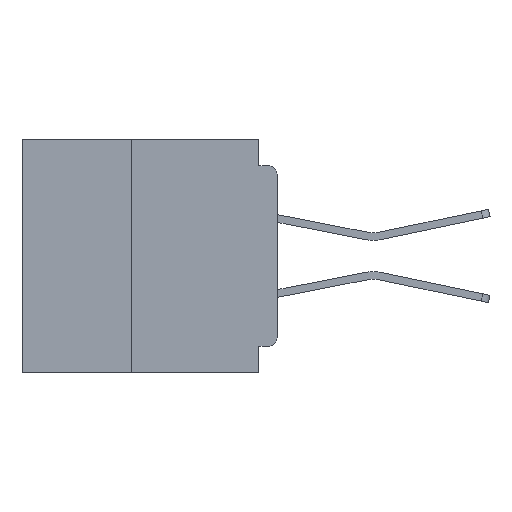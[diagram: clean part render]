
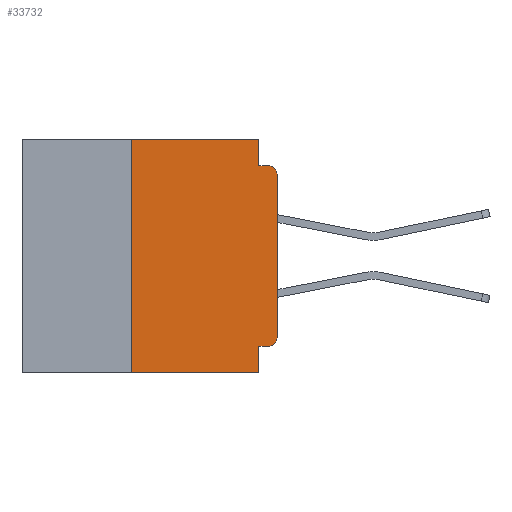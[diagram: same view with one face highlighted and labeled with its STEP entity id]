
A CAD part, left-side view. The second image highlights one B-rep face of the part: STEP entity #33732.
In plain terms, the highlighted planar face has unit normal (-1, 0, 0).
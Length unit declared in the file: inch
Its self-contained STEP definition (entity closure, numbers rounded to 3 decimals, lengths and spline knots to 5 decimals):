
#465 = CARTESIAN_POINT ( 'NONE',  ( 0., 0.437, -0.4 ) ) ;
#1967 = PLANE ( 'NONE',  #48485 ) ;
#2729 = VECTOR ( 'NONE', #35786, 39.37008 ) ;
#2895 = VECTOR ( 'NONE', #12033, 39.37008 ) ;
#3244 = VERTEX_POINT ( 'NONE', #47638 ) ;
#3533 = ORIENTED_EDGE ( 'NONE', *, *, #6978, .F. ) ;
#4077 = LINE ( 'NONE', #23876, #15611 ) ;
#4871 = VECTOR ( 'NONE', #42833, 39.37008 ) ;
#4884 = AXIS2_PLACEMENT_3D ( 'NONE', #11388, #45595, #16334 ) ;
#5886 = ORIENTED_EDGE ( 'NONE', *, *, #40494, .T. ) ;
#6628 = ORIENTED_EDGE ( 'NONE', *, *, #50341, .T. ) ;
#6978 = EDGE_CURVE ( 'NONE', #46135, #61625, #45767, .T. ) ;
#9293 = EDGE_CURVE ( 'NONE', #43562, #58347, #61376, .T. ) ;
#10098 = ORIENTED_EDGE ( 'NONE', *, *, #47548, .F. ) ;
#10456 = CARTESIAN_POINT ( 'NONE',  ( 0., 0.015, -0.06 ) ) ;
#11388 = CARTESIAN_POINT ( 'NONE',  ( 0., 0.015, -0.34 ) ) ;
#12033 = DIRECTION ( 'NONE',  ( 0., 0., 1. ) ) ;
#13224 = CARTESIAN_POINT ( 'NONE',  ( 0., 0.25, -0.4 ) ) ;
#13518 = CARTESIAN_POINT ( 'NONE',  ( 0., 0.437, 0. ) ) ;
#15385 = DIRECTION ( 'NONE',  ( 0., 0., -1. ) ) ;
#15611 = VECTOR ( 'NONE', #53480, 39.37008 ) ;
#15849 = VERTEX_POINT ( 'NONE', #16505 ) ;
#15892 = CARTESIAN_POINT ( 'NONE',  ( 0., 0.031, 0. ) ) ;
#16060 = EDGE_CURVE ( 'NONE', #26634, #33662, #48475, .T. ) ;
#16169 = CARTESIAN_POINT ( 'NONE',  ( 0., 0.25, 0. ) ) ;
#16334 = DIRECTION ( 'NONE',  ( 0., 0., -1. ) ) ;
#16505 = CARTESIAN_POINT ( 'NONE',  ( 0., 0., -0.34 ) ) ;
#17519 = LINE ( 'NONE', #55933, #2895 ) ;
#17828 = CARTESIAN_POINT ( 'NONE',  ( 0., 0.031, -0.4 ) ) ;
#18321 = CARTESIAN_POINT ( 'NONE',  ( 0., 0., -0.06 ) ) ;
#19123 = VECTOR ( 'NONE', #20232, 39.37008 ) ;
#19307 = EDGE_CURVE ( 'NONE', #15849, #43562, #17519, .T. ) ;
#20232 = DIRECTION ( 'NONE',  ( 0., -1., 0. ) ) ;
#21727 = CARTESIAN_POINT ( 'NONE',  ( 0., 0.437, 0. ) ) ;
#23099 = LINE ( 'NONE', #44211, #47508 ) ;
#23876 = CARTESIAN_POINT ( 'NONE',  ( 0., 0.031, 0. ) ) ;
#24467 = CARTESIAN_POINT ( 'NONE',  ( 0., 0.031, -0.355 ) ) ;
#25173 = ORIENTED_EDGE ( 'NONE', *, *, #19307, .T. ) ;
#25778 = ORIENTED_EDGE ( 'NONE', *, *, #30856, .F. ) ;
#26624 = DIRECTION ( 'NONE',  ( 0., 0., -1. ) ) ;
#26634 = VERTEX_POINT ( 'NONE', #57738 ) ;
#29262 = ORIENTED_EDGE ( 'NONE', *, *, #16060, .F. ) ;
#29683 = DIRECTION ( 'NONE',  ( 0., 1., 0. ) ) ;
#30856 = EDGE_CURVE ( 'NONE', #49105, #58347, #43404, .T. ) ;
#30950 = LINE ( 'NONE', #13518, #4871 ) ;
#32939 = ORIENTED_EDGE ( 'NONE', *, *, #58602, .F. ) ;
#33662 = VERTEX_POINT ( 'NONE', #16169 ) ;
#33732 = ADVANCED_FACE ( 'NONE', ( #48493 ), #1967, .F. ) ;
#33752 = EDGE_LOOP ( 'NONE', ( #25173, #57163, #25778, #10098, #32939, #29262, #5886, #3533, #45059, #6628 ) ) ;
#35786 = DIRECTION ( 'NONE',  ( 0., -1., 0. ) ) ;
#37196 = CARTESIAN_POINT ( 'NONE',  ( 0., 0.031, -0.045 ) ) ;
#37647 = DIRECTION ( 'NONE',  ( 0., 0., 1. ) ) ;
#38861 = CARTESIAN_POINT ( 'NONE',  ( 0., 0.031, -0.4 ) ) ;
#40493 = CARTESIAN_POINT ( 'NONE',  ( 0., 0., -0.045 ) ) ;
#40494 = EDGE_CURVE ( 'NONE', #26634, #61625, #45119, .T. ) ;
#42833 = DIRECTION ( 'NONE',  ( 0., -1., 0. ) ) ;
#43404 = LINE ( 'NONE', #40493, #2729 ) ;
#43562 = VERTEX_POINT ( 'NONE', #18321 ) ;
#44211 = CARTESIAN_POINT ( 'NONE',  ( 0., 0., -0.355 ) ) ;
#44470 = VERTEX_POINT ( 'NONE', #15892 ) ;
#44680 = DIRECTION ( 'NONE',  ( -1., 0., 0. ) ) ;
#45059 = ORIENTED_EDGE ( 'NONE', *, *, #49409, .F. ) ;
#45119 = LINE ( 'NONE', #465, #19123 ) ;
#45595 = DIRECTION ( 'NONE',  ( -1., 0., 0. ) ) ;
#45688 = AXIS2_PLACEMENT_3D ( 'NONE', #10456, #44680, #15385 ) ;
#45767 = LINE ( 'NONE', #17828, #61626 ) ;
#46135 = VERTEX_POINT ( 'NONE', #24467 ) ;
#47508 = VECTOR ( 'NONE', #29683, 39.37008 ) ;
#47548 = EDGE_CURVE ( 'NONE', #44470, #49105, #4077, .T. ) ;
#47638 = CARTESIAN_POINT ( 'NONE',  ( 0., 0.015, -0.355 ) ) ;
#48475 = LINE ( 'NONE', #13224, #59834 ) ;
#48485 = AXIS2_PLACEMENT_3D ( 'NONE', #21727, #55768, #26624 ) ;
#48493 = FACE_OUTER_BOUND ( 'NONE', #33752, .T. ) ;
#49105 = VERTEX_POINT ( 'NONE', #37196 ) ;
#49409 = EDGE_CURVE ( 'NONE', #3244, #46135, #23099, .T. ) ;
#50341 = EDGE_CURVE ( 'NONE', #3244, #15849, #57225, .T. ) ;
#52255 = CARTESIAN_POINT ( 'NONE',  ( 0., 0.015, -0.045 ) ) ;
#53480 = DIRECTION ( 'NONE',  ( 0., 0., -1. ) ) ;
#55768 = DIRECTION ( 'NONE',  ( 1., 0., 0. ) ) ;
#55933 = CARTESIAN_POINT ( 'NONE',  ( 0., 0., 0. ) ) ;
#56782 = DIRECTION ( 'NONE',  ( 0., 0., -1. ) ) ;
#57163 = ORIENTED_EDGE ( 'NONE', *, *, #9293, .T. ) ;
#57225 = CIRCLE ( 'NONE', #4884, 0.015 ) ;
#57738 = CARTESIAN_POINT ( 'NONE',  ( 0., 0.25, -0.4 ) ) ;
#58347 = VERTEX_POINT ( 'NONE', #52255 ) ;
#58602 = EDGE_CURVE ( 'NONE', #33662, #44470, #30950, .T. ) ;
#59834 = VECTOR ( 'NONE', #37647, 39.37008 ) ;
#61376 = CIRCLE ( 'NONE', #45688, 0.015 ) ;
#61625 = VERTEX_POINT ( 'NONE', #38861 ) ;
#61626 = VECTOR ( 'NONE', #56782, 39.37008 ) ;
